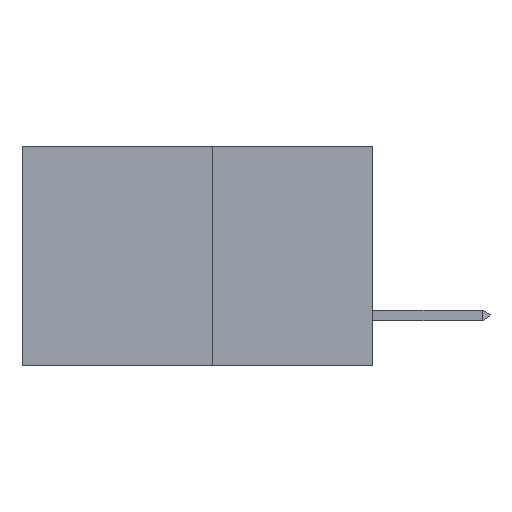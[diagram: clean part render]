
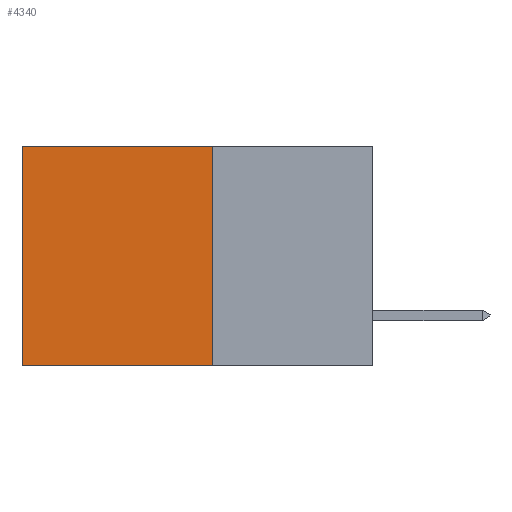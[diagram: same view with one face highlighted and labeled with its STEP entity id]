
A CAD part, left-side view. The second image highlights one B-rep face of the part: STEP entity #4340.
In plain terms, the highlighted planar face has unit normal (-1, 0, 0).
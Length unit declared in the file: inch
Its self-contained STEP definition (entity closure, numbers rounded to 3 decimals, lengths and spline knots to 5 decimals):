
#238 = LINE ( 'NONE', #7039, #1821 ) ;
#262 = VERTEX_POINT ( 'NONE', #1691 ) ;
#276 = PLANE ( 'NONE',  #8018 ) ;
#285 = EDGE_CURVE ( 'NONE', #11177, #821, #238, .T. ) ;
#410 = EDGE_CURVE ( 'NONE', #262, #1961, #5729, .T. ) ;
#821 = VERTEX_POINT ( 'NONE', #14035 ) ;
#1415 = DIRECTION ( 'NONE',  ( 0., 0., -1. ) ) ;
#1691 = CARTESIAN_POINT ( 'NONE',  ( 0.277, 0.27, -0.37 ) ) ;
#1821 = VECTOR ( 'NONE', #7992, 39.37008 ) ;
#1961 = VERTEX_POINT ( 'NONE', #4917 ) ;
#2712 = VECTOR ( 'NONE', #4014, 39.37008 ) ;
#2945 = LINE ( 'NONE', #7639, #8967 ) ;
#3378 = EDGE_CURVE ( 'NONE', #821, #1961, #2945, .T. ) ;
#3755 = ORIENTED_EDGE ( 'NONE', *, *, #410, .F. ) ;
#4014 = DIRECTION ( 'NONE',  ( 0., 1., 0. ) ) ;
#4340 = ADVANCED_FACE ( 'NONE', ( #5232 ), #276, .F. ) ;
#4917 = CARTESIAN_POINT ( 'NONE',  ( 0.277, 0.59, -0.37 ) ) ;
#4994 = CARTESIAN_POINT ( 'NONE',  ( 0.277, 0.27, -0.37 ) ) ;
#5232 = FACE_OUTER_BOUND ( 'NONE', #5733, .T. ) ;
#5729 = LINE ( 'NONE', #4994, #2712 ) ;
#5733 = EDGE_LOOP ( 'NONE', ( #12244, #3755, #10078, #13886 ) ) ;
#5874 = LINE ( 'NONE', #9011, #8194 ) ;
#7039 = CARTESIAN_POINT ( 'NONE',  ( 0.277, 0.27, 0. ) ) ;
#7056 = CARTESIAN_POINT ( 'NONE',  ( 0.277, 0.27, -0.37 ) ) ;
#7639 = CARTESIAN_POINT ( 'NONE',  ( 0.277, 0.59, -0.37 ) ) ;
#7711 = EDGE_CURVE ( 'NONE', #11177, #262, #5874, .T. ) ;
#7826 = DIRECTION ( 'NONE',  ( 0., 0., -1. ) ) ;
#7992 = DIRECTION ( 'NONE',  ( 0., 1., 0. ) ) ;
#8018 = AXIS2_PLACEMENT_3D ( 'NONE', #7056, #8225, #1415 ) ;
#8108 = CARTESIAN_POINT ( 'NONE',  ( 0.277, 0.27, 0. ) ) ;
#8194 = VECTOR ( 'NONE', #13249, 39.37008 ) ;
#8225 = DIRECTION ( 'NONE',  ( 1., 0., 0. ) ) ;
#8967 = VECTOR ( 'NONE', #7826, 39.37008 ) ;
#9011 = CARTESIAN_POINT ( 'NONE',  ( 0.277, 0.27, -0.37 ) ) ;
#10078 = ORIENTED_EDGE ( 'NONE', *, *, #7711, .F. ) ;
#11177 = VERTEX_POINT ( 'NONE', #8108 ) ;
#12244 = ORIENTED_EDGE ( 'NONE', *, *, #3378, .T. ) ;
#13249 = DIRECTION ( 'NONE',  ( 0., 0., -1. ) ) ;
#13886 = ORIENTED_EDGE ( 'NONE', *, *, #285, .T. ) ;
#14035 = CARTESIAN_POINT ( 'NONE',  ( 0.277, 0.59, 0. ) ) ;
